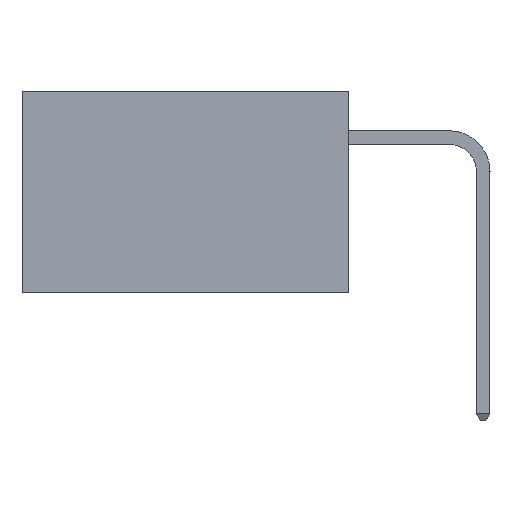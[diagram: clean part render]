
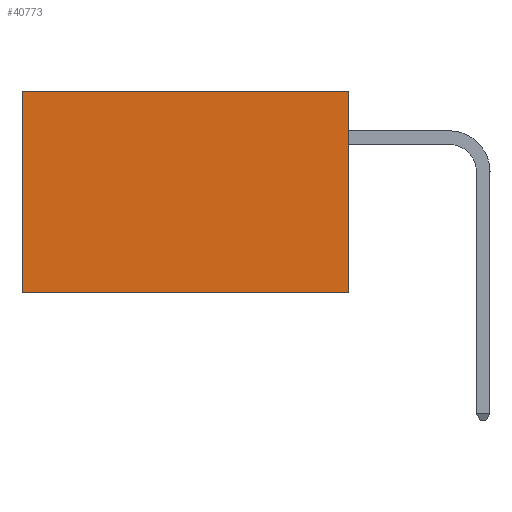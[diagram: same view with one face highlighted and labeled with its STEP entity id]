
A CAD part, left-side view. The second image highlights one B-rep face of the part: STEP entity #40773.
In plain terms, the highlighted planar face has unit normal (-1, 0, 0).
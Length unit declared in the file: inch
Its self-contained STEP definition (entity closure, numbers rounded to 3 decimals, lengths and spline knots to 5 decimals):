
#3113 = FACE_OUTER_BOUND ( 'NONE', #19697, .T. ) ;
#3504 = LINE ( 'NONE', #19277, #21365 ) ;
#3805 = VERTEX_POINT ( 'NONE', #19340 ) ;
#7899 = PLANE ( 'NONE',  #9781 ) ;
#9781 = AXIS2_PLACEMENT_3D ( 'NONE', #32717, #15078, #40052 ) ;
#12668 = DIRECTION ( 'NONE',  ( 0., 1., 0. ) ) ;
#12743 = EDGE_CURVE ( 'NONE', #3805, #16917, #20866, .T. ) ;
#12748 = DIRECTION ( 'NONE',  ( 0., 0., -1. ) ) ;
#13334 = EDGE_CURVE ( 'NONE', #40681, #36282, #3504, .T. ) ;
#13845 = ORIENTED_EDGE ( 'NONE', *, *, #13334, .T. ) ;
#15078 = DIRECTION ( 'NONE',  ( 1., 0., 0. ) ) ;
#15279 = DIRECTION ( 'NONE',  ( 0., 1., 0. ) ) ;
#16917 = VERTEX_POINT ( 'NONE', #17518 ) ;
#17518 = CARTESIAN_POINT ( 'NONE',  ( 0.2875, 0., -0.37 ) ) ;
#18486 = VECTOR ( 'NONE', #12668, 39.37008 ) ;
#19277 = CARTESIAN_POINT ( 'NONE',  ( 0.2875, 0.6, 0. ) ) ;
#19340 = CARTESIAN_POINT ( 'NONE',  ( 0.2875, 0., 0. ) ) ;
#19697 = EDGE_LOOP ( 'NONE', ( #13845, #46244, #33155, #24974 ) ) ;
#20866 = LINE ( 'NONE', #44861, #29260 ) ;
#21365 = VECTOR ( 'NONE', #22848, 39.37008 ) ;
#22848 = DIRECTION ( 'NONE',  ( 0., 0., -1. ) ) ;
#24974 = ORIENTED_EDGE ( 'NONE', *, *, #27982, .T. ) ;
#27982 = EDGE_CURVE ( 'NONE', #3805, #40681, #44680, .T. ) ;
#29260 = VECTOR ( 'NONE', #12748, 39.37008 ) ;
#32717 = CARTESIAN_POINT ( 'NONE',  ( 0.2875, 0., 0. ) ) ;
#33155 = ORIENTED_EDGE ( 'NONE', *, *, #12743, .F. ) ;
#33203 = VECTOR ( 'NONE', #15279, 39.37008 ) ;
#34041 = CARTESIAN_POINT ( 'NONE',  ( 0.2875, 0., 0. ) ) ;
#34620 = CARTESIAN_POINT ( 'NONE',  ( 0.2875, 0.6, -0.37 ) ) ;
#36282 = VERTEX_POINT ( 'NONE', #34620 ) ;
#36655 = CARTESIAN_POINT ( 'NONE',  ( 0.2875, 0., -0.37 ) ) ;
#40052 = DIRECTION ( 'NONE',  ( 0., 0., -1. ) ) ;
#40681 = VERTEX_POINT ( 'NONE', #43173 ) ;
#40773 = ADVANCED_FACE ( 'NONE', ( #3113 ), #7899, .F. ) ;
#41959 = EDGE_CURVE ( 'NONE', #16917, #36282, #43802, .T. ) ;
#43173 = CARTESIAN_POINT ( 'NONE',  ( 0.2875, 0.6, 0. ) ) ;
#43802 = LINE ( 'NONE', #36655, #33203 ) ;
#44680 = LINE ( 'NONE', #34041, #18486 ) ;
#44861 = CARTESIAN_POINT ( 'NONE',  ( 0.2875, 0., 0. ) ) ;
#46244 = ORIENTED_EDGE ( 'NONE', *, *, #41959, .F. ) ;
